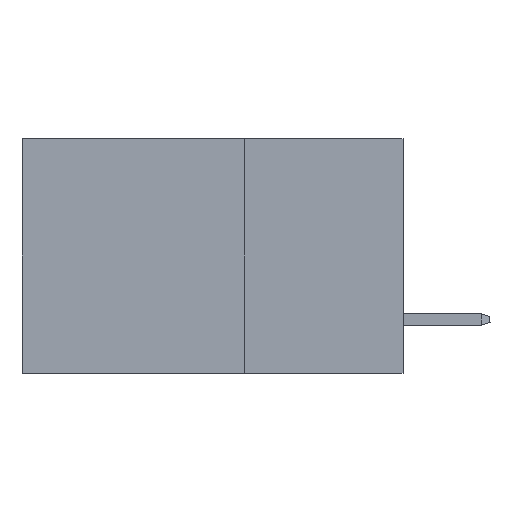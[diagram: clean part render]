
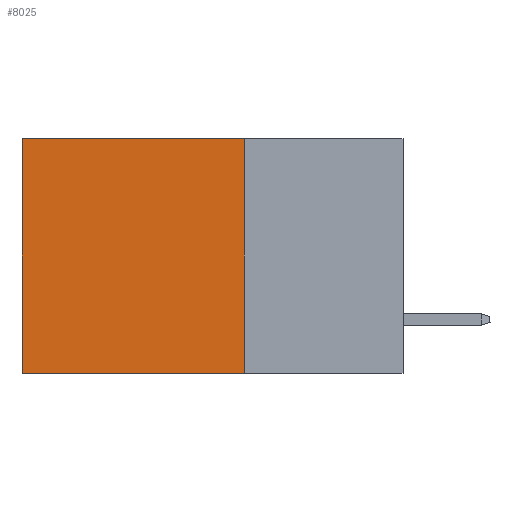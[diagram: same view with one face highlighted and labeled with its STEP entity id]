
A CAD part, left-side view. The second image highlights one B-rep face of the part: STEP entity #8025.
In plain terms, the highlighted planar face has unit normal (-1, 0, 0).
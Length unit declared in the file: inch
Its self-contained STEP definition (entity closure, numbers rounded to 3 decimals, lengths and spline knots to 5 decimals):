
#3461 = CARTESIAN_POINT ( 'NONE',  ( 0.2875, 0.6, 0. ) ) ;
#3649 = FACE_OUTER_BOUND ( 'NONE', #19751, .T. ) ;
#6573 = ORIENTED_EDGE ( 'NONE', *, *, #34443, .F. ) ;
#7096 = CARTESIAN_POINT ( 'NONE',  ( 0.2875, 0.6, -0.37 ) ) ;
#7581 = CARTESIAN_POINT ( 'NONE',  ( 0.2875, 0.25, -0.37 ) ) ;
#8025 = ADVANCED_FACE ( 'NONE', ( #3649 ), #28618, .F. ) ;
#10025 = DIRECTION ( 'NONE',  ( 1., 0., 0. ) ) ;
#11064 = CARTESIAN_POINT ( 'NONE',  ( 0.2875, 0.6, 0. ) ) ;
#12223 = VERTEX_POINT ( 'NONE', #7581 ) ;
#15387 = CARTESIAN_POINT ( 'NONE',  ( 0.2875, 0.25, -0.37 ) ) ;
#15935 = VECTOR ( 'NONE', #35358, 39.37008 ) ;
#16845 = VERTEX_POINT ( 'NONE', #7096 ) ;
#19449 = CARTESIAN_POINT ( 'NONE',  ( 0.2875, 0.25, 0. ) ) ;
#19751 = EDGE_LOOP ( 'NONE', ( #24155, #28897, #6573, #39689 ) ) ;
#24155 = ORIENTED_EDGE ( 'NONE', *, *, #28943, .T. ) ;
#24943 = DIRECTION ( 'NONE',  ( 0., 0., -1. ) ) ;
#25966 = DIRECTION ( 'NONE',  ( 0., 0., -1. ) ) ;
#26602 = DIRECTION ( 'NONE',  ( 0., 1., 0. ) ) ;
#28618 = PLANE ( 'NONE',  #35346 ) ;
#28897 = ORIENTED_EDGE ( 'NONE', *, *, #33898, .F. ) ;
#28943 = EDGE_CURVE ( 'NONE', #37120, #16845, #44545, .T. ) ;
#30315 = DIRECTION ( 'NONE',  ( 0., 1., 0. ) ) ;
#31655 = VECTOR ( 'NONE', #26602, 39.37008 ) ;
#33898 = EDGE_CURVE ( 'NONE', #12223, #16845, #34005, .T. ) ;
#34005 = LINE ( 'NONE', #15387, #47936 ) ;
#34443 = EDGE_CURVE ( 'NONE', #39221, #12223, #39504, .T. ) ;
#35346 = AXIS2_PLACEMENT_3D ( 'NONE', #43520, #10025, #24943 ) ;
#35358 = DIRECTION ( 'NONE',  ( 0., 0., -1. ) ) ;
#35780 = EDGE_CURVE ( 'NONE', #39221, #37120, #45441, .T. ) ;
#37120 = VERTEX_POINT ( 'NONE', #3461 ) ;
#37366 = CARTESIAN_POINT ( 'NONE',  ( 0.2875, 0.25, 0. ) ) ;
#38322 = VECTOR ( 'NONE', #25966, 39.37008 ) ;
#39221 = VERTEX_POINT ( 'NONE', #19449 ) ;
#39504 = LINE ( 'NONE', #42197, #15935 ) ;
#39689 = ORIENTED_EDGE ( 'NONE', *, *, #35780, .T. ) ;
#42197 = CARTESIAN_POINT ( 'NONE',  ( 0.2875, 0.25, 0. ) ) ;
#43520 = CARTESIAN_POINT ( 'NONE',  ( 0.2875, 0.25, 0. ) ) ;
#44545 = LINE ( 'NONE', #11064, #38322 ) ;
#45441 = LINE ( 'NONE', #37366, #31655 ) ;
#47936 = VECTOR ( 'NONE', #30315, 39.37008 ) ;
